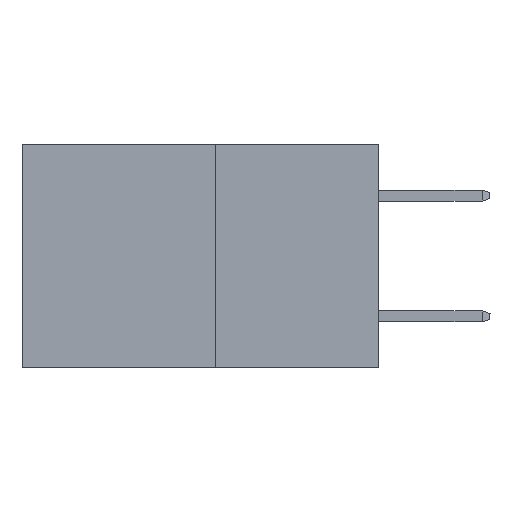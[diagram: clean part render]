
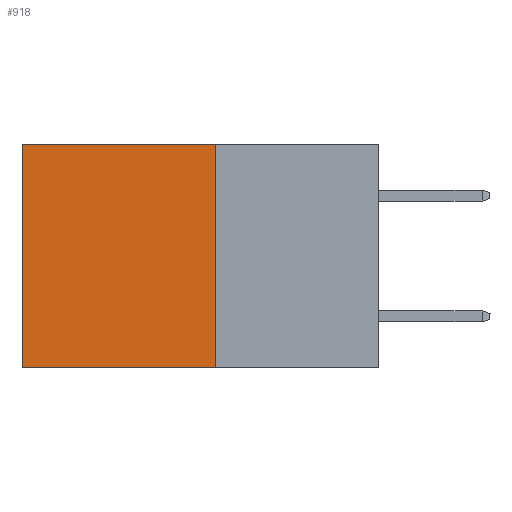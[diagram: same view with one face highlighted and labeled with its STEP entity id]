
A CAD part, left-side view. The second image highlights one B-rep face of the part: STEP entity #918.
In plain terms, the highlighted planar face has unit normal (-1, 0, 0).
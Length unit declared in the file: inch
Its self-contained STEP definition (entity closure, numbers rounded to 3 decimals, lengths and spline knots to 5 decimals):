
#435 = VECTOR ( 'NONE', #24137, 39.37008 ) ;
#529 = CARTESIAN_POINT ( 'NONE',  ( 0.277, 0.59, -0.37 ) ) ;
#918 = ADVANCED_FACE ( 'NONE', ( #2909 ), #20552, .F. ) ;
#2909 = FACE_OUTER_BOUND ( 'NONE', #10456, .T. ) ;
#3207 = CARTESIAN_POINT ( 'NONE',  ( 0.277, 0.27, -0.37 ) ) ;
#5572 = VERTEX_POINT ( 'NONE', #10239 ) ;
#5615 = VECTOR ( 'NONE', #26123, 39.37008 ) ;
#6273 = VECTOR ( 'NONE', #30186, 39.37008 ) ;
#7191 = EDGE_CURVE ( 'NONE', #11465, #5572, #24179, .T. ) ;
#7389 = DIRECTION ( 'NONE',  ( 0., 0., -1. ) ) ;
#8705 = EDGE_CURVE ( 'NONE', #11465, #25153, #12970, .T. ) ;
#9518 = CARTESIAN_POINT ( 'NONE',  ( 0.277, 0.27, -0.37 ) ) ;
#9864 = CARTESIAN_POINT ( 'NONE',  ( 0.277, 0.27, 0. ) ) ;
#9895 = VERTEX_POINT ( 'NONE', #529 ) ;
#10239 = CARTESIAN_POINT ( 'NONE',  ( 0.277, 0.59, 0. ) ) ;
#10456 = EDGE_LOOP ( 'NONE', ( #29558, #28754, #19505, #12676 ) ) ;
#11465 = VERTEX_POINT ( 'NONE', #28799 ) ;
#11639 = CARTESIAN_POINT ( 'NONE',  ( 0.277, 0.27, -0.37 ) ) ;
#12452 = LINE ( 'NONE', #11639, #6273 ) ;
#12676 = ORIENTED_EDGE ( 'NONE', *, *, #7191, .T. ) ;
#12970 = LINE ( 'NONE', #3207, #435 ) ;
#15608 = CARTESIAN_POINT ( 'NONE',  ( 0.277, 0.59, -0.37 ) ) ;
#16387 = AXIS2_PLACEMENT_3D ( 'NONE', #26586, #21967, #7389 ) ;
#17217 = VECTOR ( 'NONE', #17936, 39.37008 ) ;
#17359 = EDGE_CURVE ( 'NONE', #5572, #9895, #23340, .T. ) ;
#17936 = DIRECTION ( 'NONE',  ( 0., 0., -1. ) ) ;
#19505 = ORIENTED_EDGE ( 'NONE', *, *, #8705, .F. ) ;
#20552 = PLANE ( 'NONE',  #16387 ) ;
#21967 = DIRECTION ( 'NONE',  ( 1., 0., 0. ) ) ;
#23340 = LINE ( 'NONE', #15608, #17217 ) ;
#24137 = DIRECTION ( 'NONE',  ( 0., 0., -1. ) ) ;
#24179 = LINE ( 'NONE', #9864, #5615 ) ;
#25079 = EDGE_CURVE ( 'NONE', #25153, #9895, #12452, .T. ) ;
#25153 = VERTEX_POINT ( 'NONE', #9518 ) ;
#26123 = DIRECTION ( 'NONE',  ( 0., 1., 0. ) ) ;
#26586 = CARTESIAN_POINT ( 'NONE',  ( 0.277, 0.27, -0.37 ) ) ;
#28754 = ORIENTED_EDGE ( 'NONE', *, *, #25079, .F. ) ;
#28799 = CARTESIAN_POINT ( 'NONE',  ( 0.277, 0.27, 0. ) ) ;
#29558 = ORIENTED_EDGE ( 'NONE', *, *, #17359, .T. ) ;
#30186 = DIRECTION ( 'NONE',  ( 0., 1., 0. ) ) ;
